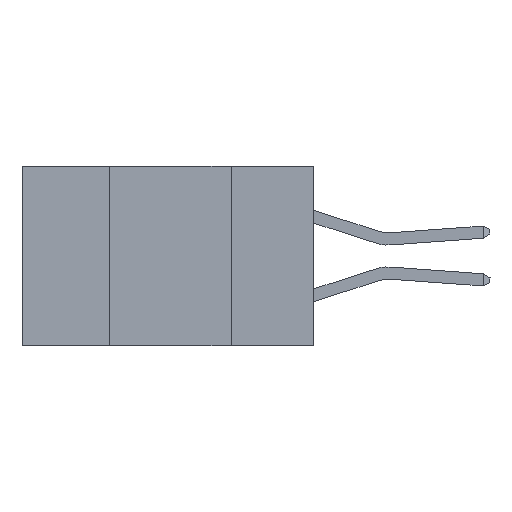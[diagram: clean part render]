
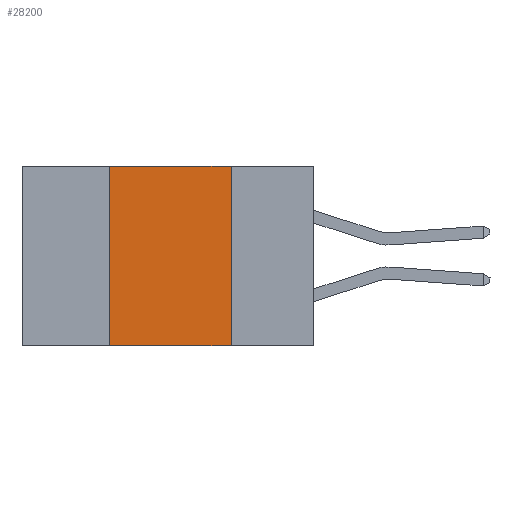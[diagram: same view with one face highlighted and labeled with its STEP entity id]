
A CAD part, left-side view. The second image highlights one B-rep face of the part: STEP entity #28200.
In plain terms, the highlighted planar face has unit normal (-1, 0, 0).
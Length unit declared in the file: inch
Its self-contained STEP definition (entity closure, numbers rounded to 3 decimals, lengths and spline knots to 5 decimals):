
#668 = DIRECTION ( 'NONE',  ( 0., 0., -1. ) ) ;
#948 = LINE ( 'NONE', #16094, #25333 ) ;
#1484 = DIRECTION ( 'NONE',  ( 0., 0., 1. ) ) ;
#2932 = VERTEX_POINT ( 'NONE', #12412 ) ;
#7877 = PLANE ( 'NONE',  #24953 ) ;
#7983 = CARTESIAN_POINT ( 'NONE',  ( 0., 0.6, 0. ) ) ;
#8140 = VERTEX_POINT ( 'NONE', #23848 ) ;
#8284 = LINE ( 'NONE', #18650, #9509 ) ;
#9131 = VERTEX_POINT ( 'NONE', #22300 ) ;
#9509 = VECTOR ( 'NONE', #668, 39.37008 ) ;
#9542 = LINE ( 'NONE', #25500, #20665 ) ;
#12240 = ORIENTED_EDGE ( 'NONE', *, *, #31920, .T. ) ;
#12412 = CARTESIAN_POINT ( 'NONE',  ( 0., 0.17, 0. ) ) ;
#12771 = ORIENTED_EDGE ( 'NONE', *, *, #15026, .F. ) ;
#12894 = CARTESIAN_POINT ( 'NONE',  ( 0., 0.42, -0.37 ) ) ;
#12907 = ORIENTED_EDGE ( 'NONE', *, *, #32112, .F. ) ;
#13205 = DIRECTION ( 'NONE',  ( 0., 0., -1. ) ) ;
#13363 = VECTOR ( 'NONE', #16568, 39.37008 ) ;
#15026 = EDGE_CURVE ( 'NONE', #31403, #8140, #948, .T. ) ;
#16094 = CARTESIAN_POINT ( 'NONE',  ( 0., 0.42, 0. ) ) ;
#16568 = DIRECTION ( 'NONE',  ( 0., -1., 0. ) ) ;
#17703 = ORIENTED_EDGE ( 'NONE', *, *, #23912, .F. ) ;
#17735 = FACE_OUTER_BOUND ( 'NONE', #29912, .T. ) ;
#18650 = CARTESIAN_POINT ( 'NONE',  ( 0., 0.17, 0. ) ) ;
#19402 = LINE ( 'NONE', #31855, #13363 ) ;
#20665 = VECTOR ( 'NONE', #22698, 39.37008 ) ;
#22300 = CARTESIAN_POINT ( 'NONE',  ( 0., 0.17, -0.37 ) ) ;
#22698 = DIRECTION ( 'NONE',  ( 0., -1., 0. ) ) ;
#23848 = CARTESIAN_POINT ( 'NONE',  ( 0., 0.42, 0. ) ) ;
#23912 = EDGE_CURVE ( 'NONE', #8140, #2932, #19402, .T. ) ;
#24953 = AXIS2_PLACEMENT_3D ( 'NONE', #7983, #30770, #13205 ) ;
#25333 = VECTOR ( 'NONE', #1484, 39.37008 ) ;
#25500 = CARTESIAN_POINT ( 'NONE',  ( 0., 0.6, -0.37 ) ) ;
#28200 = ADVANCED_FACE ( 'NONE', ( #17735 ), #7877, .F. ) ;
#29912 = EDGE_LOOP ( 'NONE', ( #12907, #17703, #12771, #12240 ) ) ;
#30770 = DIRECTION ( 'NONE',  ( 1., 0., 0. ) ) ;
#31403 = VERTEX_POINT ( 'NONE', #12894 ) ;
#31855 = CARTESIAN_POINT ( 'NONE',  ( 0., 0.6, 0. ) ) ;
#31920 = EDGE_CURVE ( 'NONE', #31403, #9131, #9542, .T. ) ;
#32112 = EDGE_CURVE ( 'NONE', #2932, #9131, #8284, .T. ) ;
